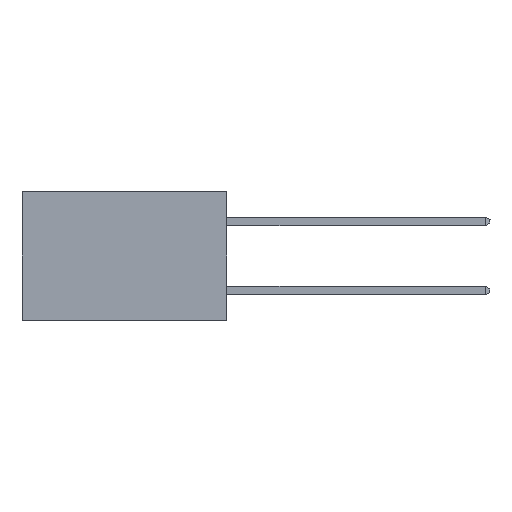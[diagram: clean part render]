
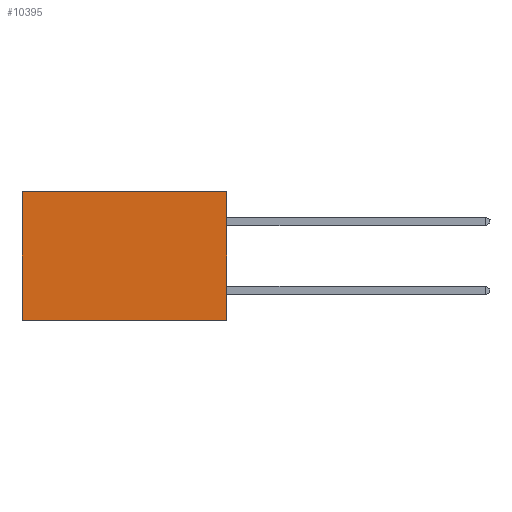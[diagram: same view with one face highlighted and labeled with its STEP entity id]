
A CAD part, left-side view. The second image highlights one B-rep face of the part: STEP entity #10395.
In plain terms, the highlighted planar face has unit normal (-1, 0, 0).
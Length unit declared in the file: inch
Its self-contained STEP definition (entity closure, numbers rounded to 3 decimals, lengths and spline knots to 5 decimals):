
#358 = DIRECTION ( 'NONE',  ( 0., 1., 0. ) ) ;
#683 = CARTESIAN_POINT ( 'NONE',  ( 0.277, 0., -0.37 ) ) ;
#1469 = CARTESIAN_POINT ( 'NONE',  ( 0.277, 0., -0.37 ) ) ;
#1802 = EDGE_CURVE ( 'NONE', #12558, #12335, #10155, .T. ) ;
#2058 = DIRECTION ( 'NONE',  ( 0., 1., 0. ) ) ;
#2083 = DIRECTION ( 'NONE',  ( 0., 0., -1. ) ) ;
#3587 = VERTEX_POINT ( 'NONE', #12505 ) ;
#3757 = LINE ( 'NONE', #13186, #17696 ) ;
#4201 = VERTEX_POINT ( 'NONE', #15259 ) ;
#6262 = CARTESIAN_POINT ( 'NONE',  ( 0.277, 0., 0. ) ) ;
#6332 = DIRECTION ( 'NONE',  ( 0., 0., -1. ) ) ;
#6365 = DIRECTION ( 'NONE',  ( 0., 0., -1. ) ) ;
#6474 = EDGE_CURVE ( 'NONE', #12335, #4201, #9810, .T. ) ;
#6512 = VECTOR ( 'NONE', #2058, 39.37008 ) ;
#6527 = VECTOR ( 'NONE', #6332, 39.37008 ) ;
#6629 = CARTESIAN_POINT ( 'NONE',  ( 0.277, 0., 0. ) ) ;
#7764 = EDGE_CURVE ( 'NONE', #3587, #4201, #3757, .T. ) ;
#7809 = EDGE_LOOP ( 'NONE', ( #17413, #12418, #11766, #12091 ) ) ;
#9004 = CARTESIAN_POINT ( 'NONE',  ( 0.277, 0., -0.37 ) ) ;
#9075 = EDGE_CURVE ( 'NONE', #12558, #3587, #13292, .T. ) ;
#9810 = LINE ( 'NONE', #683, #16510 ) ;
#10155 = LINE ( 'NONE', #1469, #6527 ) ;
#10350 = DIRECTION ( 'NONE',  ( 1., 0., 0. ) ) ;
#10395 = ADVANCED_FACE ( 'NONE', ( #16288 ), #17006, .F. ) ;
#11766 = ORIENTED_EDGE ( 'NONE', *, *, #1802, .F. ) ;
#12091 = ORIENTED_EDGE ( 'NONE', *, *, #9075, .T. ) ;
#12335 = VERTEX_POINT ( 'NONE', #15649 ) ;
#12418 = ORIENTED_EDGE ( 'NONE', *, *, #6474, .F. ) ;
#12505 = CARTESIAN_POINT ( 'NONE',  ( 0.277, 0.59, 0. ) ) ;
#12558 = VERTEX_POINT ( 'NONE', #6629 ) ;
#13186 = CARTESIAN_POINT ( 'NONE',  ( 0.277, 0.59, -0.37 ) ) ;
#13292 = LINE ( 'NONE', #6262, #6512 ) ;
#15259 = CARTESIAN_POINT ( 'NONE',  ( 0.277, 0.59, -0.37 ) ) ;
#15649 = CARTESIAN_POINT ( 'NONE',  ( 0.277, 0., -0.37 ) ) ;
#16288 = FACE_OUTER_BOUND ( 'NONE', #7809, .T. ) ;
#16510 = VECTOR ( 'NONE', #358, 39.37008 ) ;
#17006 = PLANE ( 'NONE',  #17118 ) ;
#17118 = AXIS2_PLACEMENT_3D ( 'NONE', #9004, #10350, #2083 ) ;
#17413 = ORIENTED_EDGE ( 'NONE', *, *, #7764, .T. ) ;
#17696 = VECTOR ( 'NONE', #6365, 39.37008 ) ;
